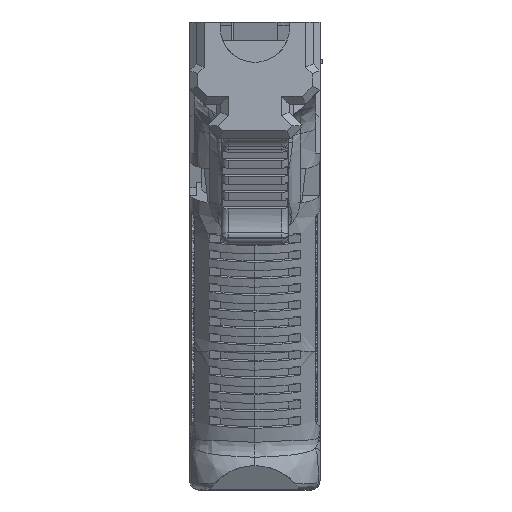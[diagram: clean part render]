
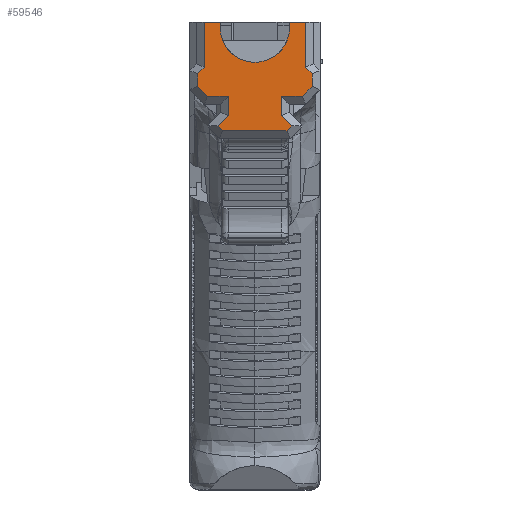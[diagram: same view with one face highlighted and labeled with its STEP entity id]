
A CAD part, left-side view. The second image highlights one B-rep face of the part: STEP entity #59546.
In plain terms, the highlighted planar face has unit normal (-1, 0, 0).
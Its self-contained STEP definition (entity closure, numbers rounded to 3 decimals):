
#8723=PLANE('',#60929);
#12115=FACE_OUTER_BOUND('',#15530,.T.);
#15530=EDGE_LOOP('',(#53552,#53553,#53554,#53555,#53556,#53557,#53558,#53559,
#53560,#53561,#53562,#53563,#53564,#53565,#53566,#53567,#53568,#53569,#53570,
#53571,#53572,#53573));
#16072=LINE('',#67589,#19737);
#19445=LINE('',#139327,#23110);
#19463=LINE('',#139368,#23128);
#19466=LINE('',#139373,#23131);
#19468=LINE('',#139377,#23133);
#19470=LINE('',#139381,#23135);
#19473=LINE('',#139386,#23138);
#19476=LINE('',#139391,#23141);
#19480=LINE('',#139401,#23145);
#19483=LINE('',#139405,#23148);
#19485=LINE('',#139409,#23150);
#19487=LINE('',#139414,#23152);
#19491=LINE('',#139420,#23156);
#19492=LINE('',#139423,#23157);
#19494=LINE('',#139427,#23159);
#19496=LINE('',#139431,#23161);
#19498=LINE('',#139434,#23163);
#19610=LINE('',#140492,#23275);
#19611=LINE('',#140494,#23276);
#19612=LINE('',#140495,#23277);
#19613=LINE('',#140496,#23278);
#19737=VECTOR('',#61117,10.);
#23110=VECTOR('',#66932,10.);
#23128=VECTOR('',#66972,10.);
#23131=VECTOR('',#66977,10.);
#23133=VECTOR('',#66981,10.);
#23135=VECTOR('',#66985,10.);
#23138=VECTOR('',#66990,10.);
#23141=VECTOR('',#66995,10.);
#23145=VECTOR('',#67005,10.);
#23148=VECTOR('',#67010,10.);
#23150=VECTOR('',#67014,10.);
#23152=VECTOR('',#67018,10.);
#23156=VECTOR('',#67024,10.);
#23157=VECTOR('',#67027,10.);
#23159=VECTOR('',#67031,10.);
#23161=VECTOR('',#67035,10.);
#23163=VECTOR('',#67039,10.);
#23275=VECTOR('',#67241,10.);
#23276=VECTOR('',#67242,10.);
#23277=VECTOR('',#67243,10.);
#23278=VECTOR('',#67244,10.);
#23553=CIRCLE('',#60859,7.765);
#23630=VERTEX_POINT('',#67586);
#23631=VERTEX_POINT('',#67588);
#29293=VERTEX_POINT('',#139319);
#29296=VERTEX_POINT('',#139325);
#29297=VERTEX_POINT('',#139329);
#29307=VERTEX_POINT('',#139366);
#29308=VERTEX_POINT('',#139367);
#29309=VERTEX_POINT('',#139372);
#29310=VERTEX_POINT('',#139376);
#29311=VERTEX_POINT('',#139380);
#29312=VERTEX_POINT('',#139385);
#29313=VERTEX_POINT('',#139389);
#29315=VERTEX_POINT('',#139399);
#29316=VERTEX_POINT('',#139400);
#29317=VERTEX_POINT('',#139407);
#29318=VERTEX_POINT('',#139411);
#29319=VERTEX_POINT('',#139413);
#29320=VERTEX_POINT('',#139418);
#29321=VERTEX_POINT('',#139422);
#29322=VERTEX_POINT('',#139426);
#29323=VERTEX_POINT('',#139430);
#29413=VERTEX_POINT('',#140493);
#29530=EDGE_CURVE('',#23631,#23630,#16072,.T.);
#38026=EDGE_CURVE('',#29296,#29293,#19445,.T.);
#38027=EDGE_CURVE('',#29297,#29296,#23553,.T.);
#38046=EDGE_CURVE('',#29307,#29308,#19463,.T.);
#38049=EDGE_CURVE('',#29309,#29307,#19466,.T.);
#38051=EDGE_CURVE('',#29310,#29309,#19468,.T.);
#38053=EDGE_CURVE('',#29311,#29310,#19470,.T.);
#38056=EDGE_CURVE('',#29312,#29311,#19473,.T.);
#38059=EDGE_CURVE('',#29308,#29313,#19476,.T.);
#38063=EDGE_CURVE('',#29315,#29316,#19480,.T.);
#38066=EDGE_CURVE('',#29313,#29315,#19483,.T.);
#38068=EDGE_CURVE('',#29316,#29317,#19485,.T.);
#38070=EDGE_CURVE('',#29318,#29319,#19487,.T.);
#38074=EDGE_CURVE('',#29320,#29318,#19491,.T.);
#38075=EDGE_CURVE('',#29317,#29321,#19492,.T.);
#38077=EDGE_CURVE('',#29321,#29322,#19494,.T.);
#38079=EDGE_CURVE('',#29322,#29323,#19496,.T.);
#38081=EDGE_CURVE('',#29323,#29320,#19498,.T.);
#38247=EDGE_CURVE('',#29319,#23630,#19610,.T.);
#38248=EDGE_CURVE('',#29413,#29312,#19611,.T.);
#38249=EDGE_CURVE('',#29413,#29293,#19612,.T.);
#38250=EDGE_CURVE('',#23631,#29297,#19613,.T.);
#53552=ORIENTED_EDGE('',*,*,#29530,.T.);
#53553=ORIENTED_EDGE('',*,*,#38247,.F.);
#53554=ORIENTED_EDGE('',*,*,#38070,.F.);
#53555=ORIENTED_EDGE('',*,*,#38074,.F.);
#53556=ORIENTED_EDGE('',*,*,#38081,.F.);
#53557=ORIENTED_EDGE('',*,*,#38079,.F.);
#53558=ORIENTED_EDGE('',*,*,#38077,.F.);
#53559=ORIENTED_EDGE('',*,*,#38075,.F.);
#53560=ORIENTED_EDGE('',*,*,#38068,.F.);
#53561=ORIENTED_EDGE('',*,*,#38063,.F.);
#53562=ORIENTED_EDGE('',*,*,#38066,.F.);
#53563=ORIENTED_EDGE('',*,*,#38059,.F.);
#53564=ORIENTED_EDGE('',*,*,#38046,.F.);
#53565=ORIENTED_EDGE('',*,*,#38049,.F.);
#53566=ORIENTED_EDGE('',*,*,#38051,.F.);
#53567=ORIENTED_EDGE('',*,*,#38053,.F.);
#53568=ORIENTED_EDGE('',*,*,#38056,.F.);
#53569=ORIENTED_EDGE('',*,*,#38248,.F.);
#53570=ORIENTED_EDGE('',*,*,#38249,.T.);
#53571=ORIENTED_EDGE('',*,*,#38026,.F.);
#53572=ORIENTED_EDGE('',*,*,#38027,.F.);
#53573=ORIENTED_EDGE('',*,*,#38250,.F.);
#59546=ADVANCED_FACE('',(#12115),#8723,.F.);
#60859=AXIS2_PLACEMENT_3D('',#139330,#66935,#66936);
#60929=AXIS2_PLACEMENT_3D('',#140491,#67239,#67240);
#61117=DIRECTION('',(0.,1.,0.));
#66932=DIRECTION('',(0.,0.,1.));
#66935=DIRECTION('center_axis',(-1.,0.,0.));
#66936=DIRECTION('ref_axis',(0.,0.,
-1.));
#66972=DIRECTION('',(0.,0.,-1.));
#66977=DIRECTION('',(0.,1.,0.));
#66981=DIRECTION('',(0.,0.707,-0.707));
#66985=DIRECTION('',(0.,0.,-1.));
#66990=DIRECTION('',(0.,-0.707,-0.707));
#66995=DIRECTION('',(0.,-0.707,-0.707));
#67005=DIRECTION('',(0.,1.,0.));
#67010=DIRECTION('',(0.,0.707,-0.707));
#67014=DIRECTION('',(0.,0.707,0.707));
#67018=DIRECTION('',(0.,-0.707,0.707));
#67024=DIRECTION('',(0.,0.,1.));
#67027=DIRECTION('',(0.,-0.707,0.707));
#67031=DIRECTION('',(0.,0.,1.));
#67035=DIRECTION('',(0.,1.,0.));
#67039=DIRECTION('',(0.,0.707,0.707));
#67239=DIRECTION('center_axis',(1.,0.,0.));
#67240=DIRECTION('ref_axis',(0.,0.,
1.));
#67241=DIRECTION('',(0.,0.,1.));
#67242=DIRECTION('',(0.,0.,-1.));
#67243=DIRECTION('',(0.,1.,0.));
#67244=DIRECTION('',(0.,0.,-1.));
#67586=CARTESIAN_POINT('',(128.368,-123.784,-24.061));
#67588=CARTESIAN_POINT('',(128.368,-127.386,-24.061));
#67589=CARTESIAN_POINT('',(128.368,-146.726,-24.061));
#139319=CARTESIAN_POINT('',(128.368,-142.914,-24.061));
#139325=CARTESIAN_POINT('',(128.368,-142.914,-25.477));
#139327=CARTESIAN_POINT('',(128.368,-142.914,-37.697));
#139329=CARTESIAN_POINT('',(128.368,-127.386,-25.477));
#139330=CARTESIAN_POINT('Origin',(128.368,-135.15,-25.35));
#139366=CARTESIAN_POINT('',(128.368,-141.086,-40.75));
#139367=CARTESIAN_POINT('',(128.368,-141.086,-45.067));
#139368=CARTESIAN_POINT('',(128.368,-141.086,-47.257));
#139372=CARTESIAN_POINT('',(128.368,-145.791,-40.75));
#139373=CARTESIAN_POINT('',(128.368,-139.114,-40.75));
#139376=CARTESIAN_POINT('',(128.368,-148.016,-38.526));
#139377=CARTESIAN_POINT('',(128.368,-142.939,-43.603));
#139380=CARTESIAN_POINT('',(128.368,-148.016,-35.672));
#139381=CARTESIAN_POINT('',(128.368,-148.016,-37.063));
#139385=CARTESIAN_POINT('',(128.368,-146.516,-34.172));
#139386=CARTESIAN_POINT('',(128.368,-150.287,-37.943));
#139389=CARTESIAN_POINT('',(128.368,-143.396,-47.377));
#139391=CARTESIAN_POINT('',(128.368,-144.5,-48.481));
#139399=CARTESIAN_POINT('',(128.368,-142.352,-48.421));
#139400=CARTESIAN_POINT('',(128.368,-127.948,-48.421));
#139401=CARTESIAN_POINT('',(128.368,-143.077,-48.421));
#139405=CARTESIAN_POINT('',(128.368,-142.551,-48.223));
#139407=CARTESIAN_POINT('',(128.368,-126.904,-47.377));
#139409=CARTESIAN_POINT('',(128.368,-131.713,-52.186));
#139411=CARTESIAN_POINT('',(128.368,-122.284,-35.672));
#139413=CARTESIAN_POINT('',(128.368,-123.784,-34.172));
#139414=CARTESIAN_POINT('',(128.368,-123.976,-33.98));
#139418=CARTESIAN_POINT('',(128.368,-122.284,-38.526));
#139420=CARTESIAN_POINT('',(128.368,-122.284,-37.063));
#139422=CARTESIAN_POINT('',(128.368,-129.214,-45.067));
#139423=CARTESIAN_POINT('',(128.368,-129.763,-44.518));
#139426=CARTESIAN_POINT('',(128.368,-129.214,-40.75));
#139427=CARTESIAN_POINT('',(128.368,-129.214,-47.257));
#139430=CARTESIAN_POINT('',(128.368,-124.509,-40.75));
#139431=CARTESIAN_POINT('',(128.368,-139.114,-40.75));
#139434=CARTESIAN_POINT('',(128.368,-131.325,-47.567));
#140491=CARTESIAN_POINT('Origin',(128.368,-143.077,-50.171));
#140492=CARTESIAN_POINT('',(128.368,-123.784,-36.809));
#140493=CARTESIAN_POINT('',(128.368,-146.516,-24.061));
#140494=CARTESIAN_POINT('',(128.368,-146.516,-36.809));
#140495=CARTESIAN_POINT('',(128.368,-146.726,-24.061));
#140496=CARTESIAN_POINT('',(128.368,-127.386,-37.697));
